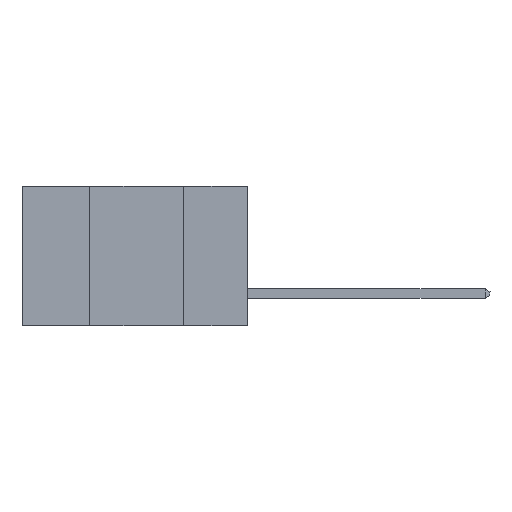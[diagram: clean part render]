
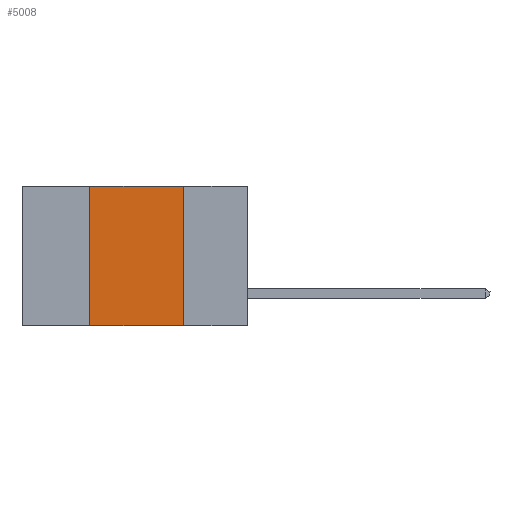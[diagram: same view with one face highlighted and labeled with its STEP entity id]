
A CAD part, left-side view. The second image highlights one B-rep face of the part: STEP entity #5008.
In plain terms, the highlighted planar face has unit normal (-1, 0, 0).
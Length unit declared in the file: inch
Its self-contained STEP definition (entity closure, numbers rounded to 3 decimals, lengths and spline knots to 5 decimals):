
#290 = CARTESIAN_POINT ( 'NONE',  ( 0., 0.6, 0. ) ) ;
#385 = ORIENTED_EDGE ( 'NONE', *, *, #10600, .F. ) ;
#1152 = DIRECTION ( 'NONE',  ( 0., -1., 0. ) ) ;
#1172 = PLANE ( 'NONE',  #8865 ) ;
#1228 = FACE_OUTER_BOUND ( 'NONE', #11210, .T. ) ;
#2152 = VECTOR ( 'NONE', #10663, 39.37008 ) ;
#3124 = ORIENTED_EDGE ( 'NONE', *, *, #11213, .F. ) ;
#3371 = LINE ( 'NONE', #5242, #2152 ) ;
#3882 = CARTESIAN_POINT ( 'NONE',  ( 0., 0.17, -0.37 ) ) ;
#4135 = LINE ( 'NONE', #7702, #6668 ) ;
#5008 = ADVANCED_FACE ( 'NONE', ( #1228 ), #1172, .F. ) ;
#5242 = CARTESIAN_POINT ( 'NONE',  ( 0., 0.42, -0.37 ) ) ;
#5358 = VECTOR ( 'NONE', #5743, 39.37008 ) ;
#5366 = ORIENTED_EDGE ( 'NONE', *, *, #10783, .T. ) ;
#5743 = DIRECTION ( 'NONE',  ( 0., 0., -1. ) ) ;
#6269 = VERTEX_POINT ( 'NONE', #9409 ) ;
#6356 = LINE ( 'NONE', #9902, #11573 ) ;
#6445 = CARTESIAN_POINT ( 'NONE',  ( 0., 0.42, 0. ) ) ;
#6514 = VERTEX_POINT ( 'NONE', #6445 ) ;
#6538 = ORIENTED_EDGE ( 'NONE', *, *, #7233, .F. ) ;
#6668 = VECTOR ( 'NONE', #11261, 39.37008 ) ;
#7233 = EDGE_CURVE ( 'NONE', #6269, #6514, #3371, .T. ) ;
#7429 = DIRECTION ( 'NONE',  ( 1., 0., 0. ) ) ;
#7702 = CARTESIAN_POINT ( 'NONE',  ( 0., 0.6, -0.37 ) ) ;
#8583 = LINE ( 'NONE', #3882, #5358 ) ;
#8865 = AXIS2_PLACEMENT_3D ( 'NONE', #290, #7429, #11042 ) ;
#9132 = VERTEX_POINT ( 'NONE', #11241 ) ;
#9409 = CARTESIAN_POINT ( 'NONE',  ( 0., 0.42, -0.37 ) ) ;
#9902 = CARTESIAN_POINT ( 'NONE',  ( 0., 0.6, 0. ) ) ;
#10180 = CARTESIAN_POINT ( 'NONE',  ( 0., 0.17, 0. ) ) ;
#10600 = EDGE_CURVE ( 'NONE', #6514, #10870, #6356, .T. ) ;
#10663 = DIRECTION ( 'NONE',  ( 0., 0., 1. ) ) ;
#10783 = EDGE_CURVE ( 'NONE', #6269, #9132, #4135, .T. ) ;
#10870 = VERTEX_POINT ( 'NONE', #10180 ) ;
#11042 = DIRECTION ( 'NONE',  ( 0., 0., -1. ) ) ;
#11210 = EDGE_LOOP ( 'NONE', ( #3124, #385, #6538, #5366 ) ) ;
#11213 = EDGE_CURVE ( 'NONE', #10870, #9132, #8583, .T. ) ;
#11241 = CARTESIAN_POINT ( 'NONE',  ( 0., 0.17, -0.37 ) ) ;
#11261 = DIRECTION ( 'NONE',  ( 0., -1., 0. ) ) ;
#11573 = VECTOR ( 'NONE', #1152, 39.37008 ) ;
